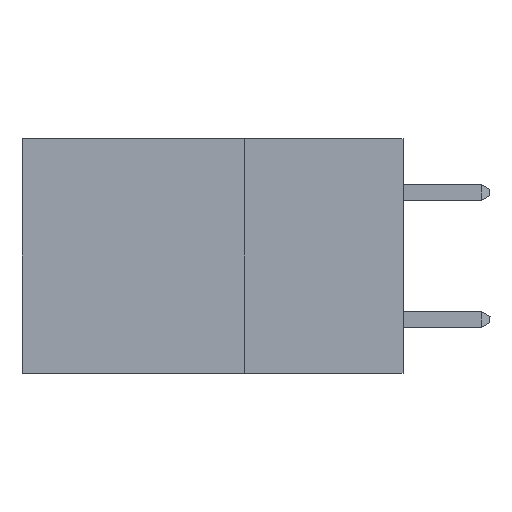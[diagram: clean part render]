
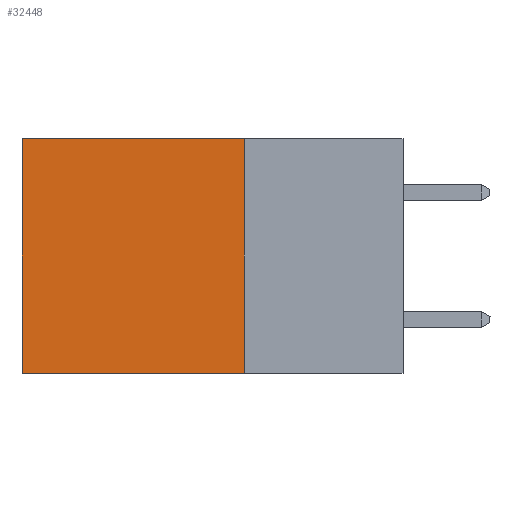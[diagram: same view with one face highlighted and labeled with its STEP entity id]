
A CAD part, left-side view. The second image highlights one B-rep face of the part: STEP entity #32448.
In plain terms, the highlighted planar face has unit normal (-1, 0, 0).
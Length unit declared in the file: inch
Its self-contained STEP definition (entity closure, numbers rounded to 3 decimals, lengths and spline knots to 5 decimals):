
#1800 = CARTESIAN_POINT ( 'NONE',  ( 0.2875, 0.25, -0.37 ) ) ;
#1862 = EDGE_CURVE ( 'NONE', #16709, #18862, #32656, .T. ) ;
#2137 = DIRECTION ( 'NONE',  ( 0., 0., -1. ) ) ;
#4001 = LINE ( 'NONE', #4636, #36896 ) ;
#4260 = EDGE_CURVE ( 'NONE', #16709, #14738, #34277, .T. ) ;
#4636 = CARTESIAN_POINT ( 'NONE',  ( 0.2875, 0.6, 0. ) ) ;
#5303 = CARTESIAN_POINT ( 'NONE',  ( 0.2875, 0.25, 0. ) ) ;
#6196 = VERTEX_POINT ( 'NONE', #7547 ) ;
#7547 = CARTESIAN_POINT ( 'NONE',  ( 0.2875, 0.6, -0.37 ) ) ;
#9800 = CARTESIAN_POINT ( 'NONE',  ( 0.2875, 0.25, -0.37 ) ) ;
#10249 = ORIENTED_EDGE ( 'NONE', *, *, #17523, .F. ) ;
#14738 = VERTEX_POINT ( 'NONE', #9800 ) ;
#16709 = VERTEX_POINT ( 'NONE', #39201 ) ;
#17523 = EDGE_CURVE ( 'NONE', #14738, #6196, #18424, .T. ) ;
#18424 = LINE ( 'NONE', #1800, #22990 ) ;
#18862 = VERTEX_POINT ( 'NONE', #19100 ) ;
#19100 = CARTESIAN_POINT ( 'NONE',  ( 0.2875, 0.6, 0. ) ) ;
#19208 = CARTESIAN_POINT ( 'NONE',  ( 0.2875, 0.25, 0. ) ) ;
#19390 = ORIENTED_EDGE ( 'NONE', *, *, #39487, .T. ) ;
#20305 = VECTOR ( 'NONE', #22631, 39.37008 ) ;
#20858 = DIRECTION ( 'NONE',  ( 0., 0., -1. ) ) ;
#22102 = PLANE ( 'NONE',  #40184 ) ;
#22631 = DIRECTION ( 'NONE',  ( 0., 1., 0. ) ) ;
#22990 = VECTOR ( 'NONE', #35767, 39.37008 ) ;
#26966 = DIRECTION ( 'NONE',  ( 0., 0., -1. ) ) ;
#28019 = ORIENTED_EDGE ( 'NONE', *, *, #1862, .T. ) ;
#28878 = VECTOR ( 'NONE', #26966, 39.37008 ) ;
#32448 = ADVANCED_FACE ( 'NONE', ( #38980 ), #22102, .F. ) ;
#32481 = EDGE_LOOP ( 'NONE', ( #19390, #10249, #43360, #28019 ) ) ;
#32568 = DIRECTION ( 'NONE',  ( 1., 0., 0. ) ) ;
#32656 = LINE ( 'NONE', #5303, #20305 ) ;
#33625 = CARTESIAN_POINT ( 'NONE',  ( 0.2875, 0.25, 0. ) ) ;
#34277 = LINE ( 'NONE', #33625, #28878 ) ;
#35767 = DIRECTION ( 'NONE',  ( 0., 1., 0. ) ) ;
#36896 = VECTOR ( 'NONE', #20858, 39.37008 ) ;
#38980 = FACE_OUTER_BOUND ( 'NONE', #32481, .T. ) ;
#39201 = CARTESIAN_POINT ( 'NONE',  ( 0.2875, 0.25, 0. ) ) ;
#39487 = EDGE_CURVE ( 'NONE', #18862, #6196, #4001, .T. ) ;
#40184 = AXIS2_PLACEMENT_3D ( 'NONE', #19208, #32568, #2137 ) ;
#43360 = ORIENTED_EDGE ( 'NONE', *, *, #4260, .F. ) ;
